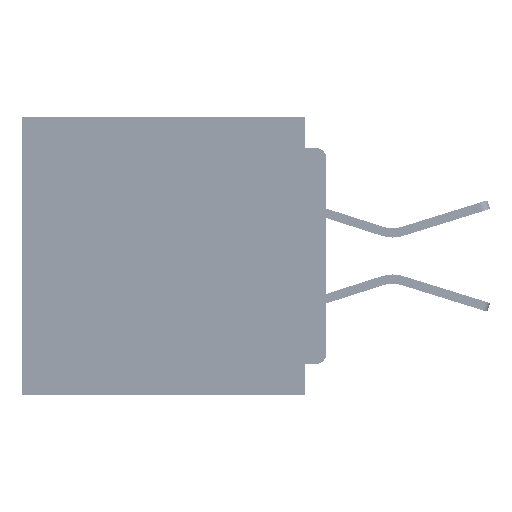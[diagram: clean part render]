
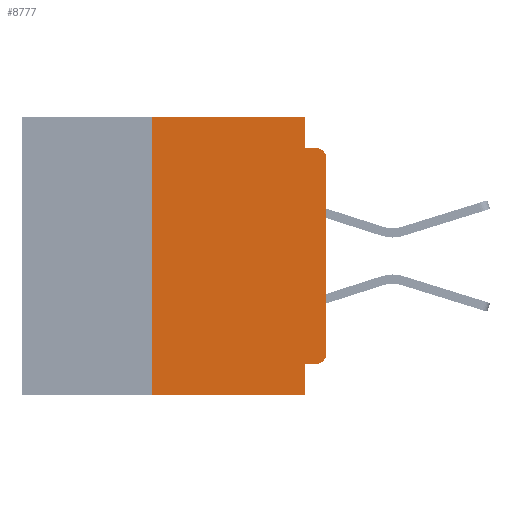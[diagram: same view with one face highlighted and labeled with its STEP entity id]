
A CAD part, left-side view. The second image highlights one B-rep face of the part: STEP entity #8777.
In plain terms, the highlighted planar face has unit normal (-1, 0, 0).
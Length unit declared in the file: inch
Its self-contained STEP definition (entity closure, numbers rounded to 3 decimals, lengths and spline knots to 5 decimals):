
#1040 = CARTESIAN_POINT ( 'NONE',  ( 0., 0.437, 0. ) ) ;
#2483 = EDGE_CURVE ( 'NONE', #63714, #46713, #36719, .T. ) ;
#4059 = CARTESIAN_POINT ( 'NONE',  ( 0., 0., -0.34 ) ) ;
#4687 = VECTOR ( 'NONE', #40810, 39.37008 ) ;
#5308 = DIRECTION ( 'NONE',  ( -1., 0., 0. ) ) ;
#7014 = EDGE_CURVE ( 'NONE', #28725, #18768, #44498, .T. ) ;
#8146 = DIRECTION ( 'NONE',  ( 1., 0., 0. ) ) ;
#8777 = ADVANCED_FACE ( 'NONE', ( #63707 ), #40235, .F. ) ;
#9630 = CARTESIAN_POINT ( 'NONE',  ( 0., 0., -0.06 ) ) ;
#11249 = CARTESIAN_POINT ( 'NONE',  ( 0., 0., 0. ) ) ;
#11314 = ORIENTED_EDGE ( 'NONE', *, *, #20744, .F. ) ;
#15407 = AXIS2_PLACEMENT_3D ( 'NONE', #37469, #5308, #42816 ) ;
#15524 = ORIENTED_EDGE ( 'NONE', *, *, #36303, .F. ) ;
#15641 = DIRECTION ( 'NONE',  ( -1., 0., 0. ) ) ;
#16634 = DIRECTION ( 'NONE',  ( 0., 0., 1. ) ) ;
#18751 = CARTESIAN_POINT ( 'NONE',  ( 0., 0.437, 0. ) ) ;
#18768 = VERTEX_POINT ( 'NONE', #21340 ) ;
#19010 = LINE ( 'NONE', #45921, #4687 ) ;
#20744 = EDGE_CURVE ( 'NONE', #30492, #48522, #22799, .T. ) ;
#20867 = CARTESIAN_POINT ( 'NONE',  ( 0., 0.437, -0.4 ) ) ;
#21340 = CARTESIAN_POINT ( 'NONE',  ( 0., 0.031, -0.4 ) ) ;
#22799 = LINE ( 'NONE', #1040, #49501 ) ;
#23476 = CARTESIAN_POINT ( 'NONE',  ( 0., 0.25, 0. ) ) ;
#23753 = VERTEX_POINT ( 'NONE', #9630 ) ;
#25514 = ORIENTED_EDGE ( 'NONE', *, *, #7014, .T. ) ;
#26805 = EDGE_CURVE ( 'NONE', #28725, #30492, #57791, .T. ) ;
#28725 = VERTEX_POINT ( 'NONE', #36692 ) ;
#29266 = CARTESIAN_POINT ( 'NONE',  ( 0., 0.015, -0.045 ) ) ;
#29351 = CARTESIAN_POINT ( 'NONE',  ( 0., 0.25, -0.4 ) ) ;
#30492 = VERTEX_POINT ( 'NONE', #23476 ) ;
#30878 = CARTESIAN_POINT ( 'NONE',  ( 0., 0.031, -0.355 ) ) ;
#33063 = EDGE_CURVE ( 'NONE', #48522, #63714, #57689, .T. ) ;
#33075 = ORIENTED_EDGE ( 'NONE', *, *, #33063, .F. ) ;
#33907 = VERTEX_POINT ( 'NONE', #4059 ) ;
#34019 = ORIENTED_EDGE ( 'NONE', *, *, #2483, .F. ) ;
#34699 = DIRECTION ( 'NONE',  ( 0., 0., 1. ) ) ;
#35511 = CARTESIAN_POINT ( 'NONE',  ( 0., 0.031, 0. ) ) ;
#36197 = CARTESIAN_POINT ( 'NONE',  ( 0., 0.031, -0.4 ) ) ;
#36303 = EDGE_CURVE ( 'NONE', #50536, #18768, #53631, .T. ) ;
#36692 = CARTESIAN_POINT ( 'NONE',  ( 0., 0.25, -0.4 ) ) ;
#36719 = LINE ( 'NONE', #42353, #65023 ) ;
#37469 = CARTESIAN_POINT ( 'NONE',  ( 0., 0.015, -0.06 ) ) ;
#39228 = CIRCLE ( 'NONE', #15407, 0.015 ) ;
#39453 = VERTEX_POINT ( 'NONE', #41686 ) ;
#39755 = ORIENTED_EDGE ( 'NONE', *, *, #51856, .T. ) ;
#40235 = PLANE ( 'NONE',  #58007 ) ;
#40810 = DIRECTION ( 'NONE',  ( 0., 1., 0. ) ) ;
#41686 = CARTESIAN_POINT ( 'NONE',  ( 0., 0.015, -0.355 ) ) ;
#42353 = CARTESIAN_POINT ( 'NONE',  ( 0., 0., -0.045 ) ) ;
#42768 = EDGE_CURVE ( 'NONE', #33907, #23753, #63979, .T. ) ;
#42816 = DIRECTION ( 'NONE',  ( 0., 0., -1. ) ) ;
#43499 = VECTOR ( 'NONE', #65886, 39.37008 ) ;
#44498 = LINE ( 'NONE', #20867, #57009 ) ;
#45248 = VECTOR ( 'NONE', #34699, 39.37008 ) ;
#45612 = DIRECTION ( 'NONE',  ( 0., 0., -1. ) ) ;
#45921 = CARTESIAN_POINT ( 'NONE',  ( 0., 0., -0.355 ) ) ;
#46460 = VECTOR ( 'NONE', #16634, 39.37008 ) ;
#46667 = DIRECTION ( 'NONE',  ( 0., 0., -1. ) ) ;
#46713 = VERTEX_POINT ( 'NONE', #29266 ) ;
#47666 = CARTESIAN_POINT ( 'NONE',  ( 0., 0.015, -0.34 ) ) ;
#48392 = DIRECTION ( 'NONE',  ( 0., -1., 0. ) ) ;
#48522 = VERTEX_POINT ( 'NONE', #35511 ) ;
#49501 = VECTOR ( 'NONE', #54704, 39.37008 ) ;
#50536 = VERTEX_POINT ( 'NONE', #30878 ) ;
#51856 = EDGE_CURVE ( 'NONE', #23753, #46713, #39228, .T. ) ;
#53073 = DIRECTION ( 'NONE',  ( 0., 0., -1. ) ) ;
#53093 = ORIENTED_EDGE ( 'NONE', *, *, #42768, .T. ) ;
#53631 = LINE ( 'NONE', #36197, #66059 ) ;
#54019 = ORIENTED_EDGE ( 'NONE', *, *, #26805, .F. ) ;
#54506 = CARTESIAN_POINT ( 'NONE',  ( 0., 0.031, -0.045 ) ) ;
#54704 = DIRECTION ( 'NONE',  ( 0., -1., 0. ) ) ;
#56995 = EDGE_CURVE ( 'NONE', #39453, #50536, #19010, .T. ) ;
#57009 = VECTOR ( 'NONE', #63544, 39.37008 ) ;
#57492 = ORIENTED_EDGE ( 'NONE', *, *, #64046, .T. ) ;
#57689 = LINE ( 'NONE', #60581, #43499 ) ;
#57791 = LINE ( 'NONE', #29351, #45248 ) ;
#58007 = AXIS2_PLACEMENT_3D ( 'NONE', #18751, #8146, #45612 ) ;
#60581 = CARTESIAN_POINT ( 'NONE',  ( 0., 0.031, 0. ) ) ;
#62380 = ORIENTED_EDGE ( 'NONE', *, *, #56995, .F. ) ;
#63544 = DIRECTION ( 'NONE',  ( 0., -1., 0. ) ) ;
#63707 = FACE_OUTER_BOUND ( 'NONE', #66680, .T. ) ;
#63714 = VERTEX_POINT ( 'NONE', #54506 ) ;
#63979 = LINE ( 'NONE', #11249, #46460 ) ;
#64046 = EDGE_CURVE ( 'NONE', #39453, #33907, #64101, .T. ) ;
#64101 = CIRCLE ( 'NONE', #66911, 0.015 ) ;
#65023 = VECTOR ( 'NONE', #48392, 39.37008 ) ;
#65886 = DIRECTION ( 'NONE',  ( 0., 0., -1. ) ) ;
#66059 = VECTOR ( 'NONE', #46667, 39.37008 ) ;
#66680 = EDGE_LOOP ( 'NONE', ( #53093, #39755, #34019, #33075, #11314, #54019, #25514, #15524, #62380, #57492 ) ) ;
#66911 = AXIS2_PLACEMENT_3D ( 'NONE', #47666, #15641, #53073 ) ;
